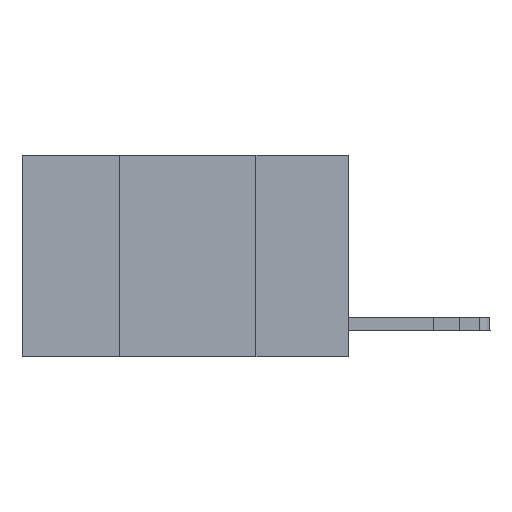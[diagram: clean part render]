
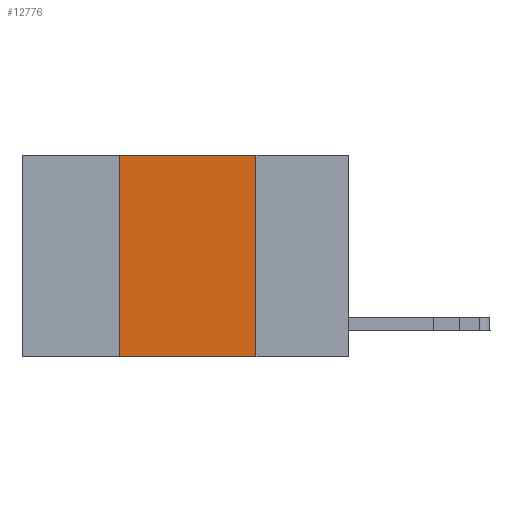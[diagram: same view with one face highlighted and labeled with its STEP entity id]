
A CAD part, left-side view. The second image highlights one B-rep face of the part: STEP entity #12776.
In plain terms, the highlighted planar face has unit normal (-1, 0, 0).
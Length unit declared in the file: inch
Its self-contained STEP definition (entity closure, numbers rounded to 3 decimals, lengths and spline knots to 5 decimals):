
#705 = CARTESIAN_POINT ( 'NONE',  ( 0., 0.6, -0.37 ) ) ;
#764 = VECTOR ( 'NONE', #15520, 39.37008 ) ;
#2100 = ORIENTED_EDGE ( 'NONE', *, *, #3162, .T. ) ;
#2265 = LINE ( 'NONE', #11909, #10949 ) ;
#2380 = CARTESIAN_POINT ( 'NONE',  ( 0., 0.17, -0.37 ) ) ;
#2758 = DIRECTION ( 'NONE',  ( 0., -1., 0. ) ) ;
#3162 = EDGE_CURVE ( 'NONE', #4770, #13276, #14108, .T. ) ;
#3240 = CARTESIAN_POINT ( 'NONE',  ( 0., 0.42, 0. ) ) ;
#4584 = VERTEX_POINT ( 'NONE', #10855 ) ;
#4770 = VERTEX_POINT ( 'NONE', #19779 ) ;
#4882 = ORIENTED_EDGE ( 'NONE', *, *, #8532, .F. ) ;
#4987 = DIRECTION ( 'NONE',  ( 0., 0., -1. ) ) ;
#5188 = CARTESIAN_POINT ( 'NONE',  ( 0., 0.6, 0. ) ) ;
#5458 = DIRECTION ( 'NONE',  ( 0., 0., 1. ) ) ;
#5608 = VERTEX_POINT ( 'NONE', #3240 ) ;
#6788 = PLANE ( 'NONE',  #8557 ) ;
#7175 = ORIENTED_EDGE ( 'NONE', *, *, #12085, .F. ) ;
#8532 = EDGE_CURVE ( 'NONE', #4770, #5608, #2265, .T. ) ;
#8557 = AXIS2_PLACEMENT_3D ( 'NONE', #5188, #11741, #4987 ) ;
#8895 = DIRECTION ( 'NONE',  ( 0., 0., -1. ) ) ;
#10153 = VECTOR ( 'NONE', #8895, 39.37008 ) ;
#10747 = VECTOR ( 'NONE', #2758, 39.37008 ) ;
#10855 = CARTESIAN_POINT ( 'NONE',  ( 0., 0.17, 0. ) ) ;
#10949 = VECTOR ( 'NONE', #5458, 39.37008 ) ;
#11741 = DIRECTION ( 'NONE',  ( 1., 0., 0. ) ) ;
#11909 = CARTESIAN_POINT ( 'NONE',  ( 0., 0.42, 0. ) ) ;
#12085 = EDGE_CURVE ( 'NONE', #4584, #13276, #17296, .T. ) ;
#12569 = EDGE_LOOP ( 'NONE', ( #7175, #13591, #4882, #2100 ) ) ;
#12776 = ADVANCED_FACE ( 'NONE', ( #16377 ), #6788, .F. ) ;
#13276 = VERTEX_POINT ( 'NONE', #2380 ) ;
#13591 = ORIENTED_EDGE ( 'NONE', *, *, #21036, .F. ) ;
#14108 = LINE ( 'NONE', #705, #764 ) ;
#15520 = DIRECTION ( 'NONE',  ( 0., -1., 0. ) ) ;
#16377 = FACE_OUTER_BOUND ( 'NONE', #12569, .T. ) ;
#17296 = LINE ( 'NONE', #18782, #10153 ) ;
#18782 = CARTESIAN_POINT ( 'NONE',  ( 0., 0.17, 0. ) ) ;
#19064 = LINE ( 'NONE', #21108, #10747 ) ;
#19779 = CARTESIAN_POINT ( 'NONE',  ( 0., 0.42, -0.37 ) ) ;
#21036 = EDGE_CURVE ( 'NONE', #5608, #4584, #19064, .T. ) ;
#21108 = CARTESIAN_POINT ( 'NONE',  ( 0., 0.6, 0. ) ) ;
